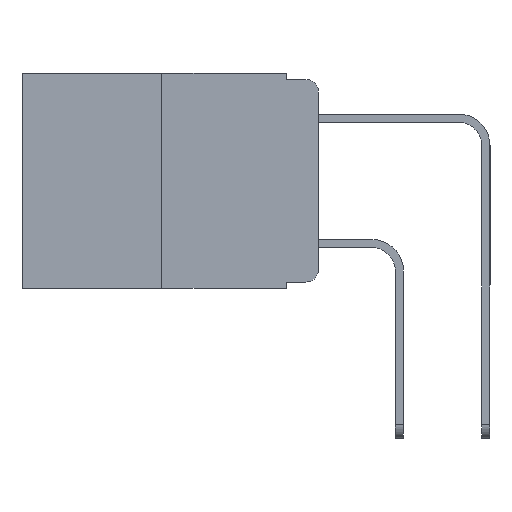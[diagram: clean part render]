
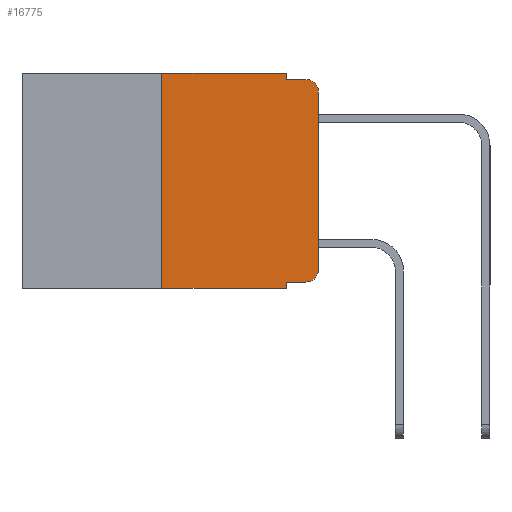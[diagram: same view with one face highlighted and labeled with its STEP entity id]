
A CAD part, left-side view. The second image highlights one B-rep face of the part: STEP entity #16775.
In plain terms, the highlighted planar face has unit normal (-1, 0, 0).
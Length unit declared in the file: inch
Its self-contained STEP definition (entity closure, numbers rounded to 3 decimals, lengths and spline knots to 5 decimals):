
#349 = CARTESIAN_POINT ( 'NONE',  ( 0., 0.25, 0. ) ) ;
#441 = CARTESIAN_POINT ( 'NONE',  ( 0., 0.02, -0.333 ) ) ;
#443 = VECTOR ( 'NONE', #15341, 39.37008 ) ;
#515 = ORIENTED_EDGE ( 'NONE', *, *, #9326, .F. ) ;
#640 = AXIS2_PLACEMENT_3D ( 'NONE', #11628, #3157, #12953 ) ;
#671 = AXIS2_PLACEMENT_3D ( 'NONE', #4486, #14166, #5902 ) ;
#764 = EDGE_CURVE ( 'NONE', #14089, #13133, #11071, .T. ) ;
#1263 = DIRECTION ( 'NONE',  ( 0., -1., 0. ) ) ;
#1606 = VERTEX_POINT ( 'NONE', #5607 ) ;
#1990 = CIRCLE ( 'NONE', #640, 0.02 ) ;
#2252 = ORIENTED_EDGE ( 'NONE', *, *, #8366, .F. ) ;
#2493 = ORIENTED_EDGE ( 'NONE', *, *, #13398, .F. ) ;
#2664 = CARTESIAN_POINT ( 'NONE',  ( 0., 0.473, 0. ) ) ;
#2732 = DIRECTION ( 'NONE',  ( 0., 0., -1. ) ) ;
#2929 = DIRECTION ( 'NONE',  ( 0., 0., -1. ) ) ;
#3157 = DIRECTION ( 'NONE',  ( -1., 0., 0. ) ) ;
#3510 = CIRCLE ( 'NONE', #671, 0.02 ) ;
#3553 = CARTESIAN_POINT ( 'NONE',  ( 0., 0.051, -0.01 ) ) ;
#3630 = VERTEX_POINT ( 'NONE', #11614 ) ;
#4084 = EDGE_CURVE ( 'NONE', #12914, #17762, #10763, .T. ) ;
#4170 = VECTOR ( 'NONE', #10276, 39.37008 ) ;
#4221 = CARTESIAN_POINT ( 'NONE',  ( 0., 0.051, -0.01 ) ) ;
#4344 = LINE ( 'NONE', #13959, #443 ) ;
#4486 = CARTESIAN_POINT ( 'NONE',  ( 0., 0.02, -0.03 ) ) ;
#4507 = CARTESIAN_POINT ( 'NONE',  ( 0., 0.25, -0.343 ) ) ;
#4748 = LINE ( 'NONE', #11322, #11327 ) ;
#5154 = ORIENTED_EDGE ( 'NONE', *, *, #4084, .F. ) ;
#5607 = CARTESIAN_POINT ( 'NONE',  ( 0., 0.051, 0. ) ) ;
#5687 = DIRECTION ( 'NONE',  ( 0., 0., 1. ) ) ;
#5902 = DIRECTION ( 'NONE',  ( 0., 0., -1. ) ) ;
#6348 = ORIENTED_EDGE ( 'NONE', *, *, #17385, .T. ) ;
#6598 = VERTEX_POINT ( 'NONE', #8873 ) ;
#6816 = DIRECTION ( 'NONE',  ( 0., -1., 0. ) ) ;
#6916 = CARTESIAN_POINT ( 'NONE',  ( 0., 0.051, -0.343 ) ) ;
#7031 = CARTESIAN_POINT ( 'NONE',  ( 0., 0.02, -0.01 ) ) ;
#7426 = VECTOR ( 'NONE', #10421, 39.37008 ) ;
#7530 = ORIENTED_EDGE ( 'NONE', *, *, #10831, .T. ) ;
#7850 = VERTEX_POINT ( 'NONE', #15649 ) ;
#8357 = ORIENTED_EDGE ( 'NONE', *, *, #764, .F. ) ;
#8366 = EDGE_CURVE ( 'NONE', #7850, #1606, #4344, .T. ) ;
#8481 = VECTOR ( 'NONE', #6816, 39.37008 ) ;
#8873 = CARTESIAN_POINT ( 'NONE',  ( 0., 0., -0.313 ) ) ;
#8878 = CARTESIAN_POINT ( 'NONE',  ( 0., 0.051, 0. ) ) ;
#9326 = EDGE_CURVE ( 'NONE', #16812, #7850, #14738, .T. ) ;
#9416 = CARTESIAN_POINT ( 'NONE',  ( 0., 0.051, 0. ) ) ;
#9645 = DIRECTION ( 'NONE',  ( 0., -1., 0. ) ) ;
#9825 = VECTOR ( 'NONE', #9645, 39.37008 ) ;
#10276 = DIRECTION ( 'NONE',  ( 0., 0., -1. ) ) ;
#10421 = DIRECTION ( 'NONE',  ( 0., 0., 1. ) ) ;
#10498 = CARTESIAN_POINT ( 'NONE',  ( 0., 0.051, -0.333 ) ) ;
#10763 = LINE ( 'NONE', #4221, #17556 ) ;
#10831 = EDGE_CURVE ( 'NONE', #16812, #13133, #15738, .T. ) ;
#11071 = LINE ( 'NONE', #9416, #12357 ) ;
#11197 = DIRECTION ( 'NONE',  ( 1., 0., 0. ) ) ;
#11322 = CARTESIAN_POINT ( 'NONE',  ( 0., 0., 0. ) ) ;
#11327 = VECTOR ( 'NONE', #5687, 39.37008 ) ;
#11614 = CARTESIAN_POINT ( 'NONE',  ( 0., 0., -0.03 ) ) ;
#11628 = CARTESIAN_POINT ( 'NONE',  ( 0., 0.02, -0.313 ) ) ;
#12350 = ORIENTED_EDGE ( 'NONE', *, *, #14993, .T. ) ;
#12357 = VECTOR ( 'NONE', #2929, 39.37008 ) ;
#12914 = VERTEX_POINT ( 'NONE', #3553 ) ;
#12953 = DIRECTION ( 'NONE',  ( 0., 0., -1. ) ) ;
#13133 = VERTEX_POINT ( 'NONE', #6916 ) ;
#13398 = EDGE_CURVE ( 'NONE', #1606, #12914, #15214, .T. ) ;
#13655 = CARTESIAN_POINT ( 'NONE',  ( 0., 0.051, -0.333 ) ) ;
#13959 = CARTESIAN_POINT ( 'NONE',  ( 0., 0.473, 0. ) ) ;
#14089 = VERTEX_POINT ( 'NONE', #10498 ) ;
#14166 = DIRECTION ( 'NONE',  ( -1., 0., 0. ) ) ;
#14738 = LINE ( 'NONE', #349, #7426 ) ;
#14882 = EDGE_CURVE ( 'NONE', #14089, #18022, #17055, .T. ) ;
#14993 = EDGE_CURVE ( 'NONE', #6598, #3630, #4748, .T. ) ;
#15054 = CARTESIAN_POINT ( 'NONE',  ( 0., 0.473, -0.343 ) ) ;
#15118 = EDGE_CURVE ( 'NONE', #18022, #6598, #1990, .T. ) ;
#15214 = LINE ( 'NONE', #8878, #4170 ) ;
#15341 = DIRECTION ( 'NONE',  ( 0., -1., 0. ) ) ;
#15649 = CARTESIAN_POINT ( 'NONE',  ( 0., 0.25, 0. ) ) ;
#15738 = LINE ( 'NONE', #15054, #8481 ) ;
#15810 = AXIS2_PLACEMENT_3D ( 'NONE', #2664, #11197, #2732 ) ;
#16438 = EDGE_LOOP ( 'NONE', ( #12350, #6348, #5154, #2493, #2252, #515, #7530, #8357, #16702, #16910 ) ) ;
#16588 = PLANE ( 'NONE',  #15810 ) ;
#16702 = ORIENTED_EDGE ( 'NONE', *, *, #14882, .T. ) ;
#16775 = ADVANCED_FACE ( 'NONE', ( #17616 ), #16588, .F. ) ;
#16812 = VERTEX_POINT ( 'NONE', #4507 ) ;
#16910 = ORIENTED_EDGE ( 'NONE', *, *, #15118, .T. ) ;
#17055 = LINE ( 'NONE', #13655, #9825 ) ;
#17385 = EDGE_CURVE ( 'NONE', #3630, #17762, #3510, .T. ) ;
#17556 = VECTOR ( 'NONE', #1263, 39.37008 ) ;
#17616 = FACE_OUTER_BOUND ( 'NONE', #16438, .T. ) ;
#17762 = VERTEX_POINT ( 'NONE', #7031 ) ;
#18022 = VERTEX_POINT ( 'NONE', #441 ) ;
